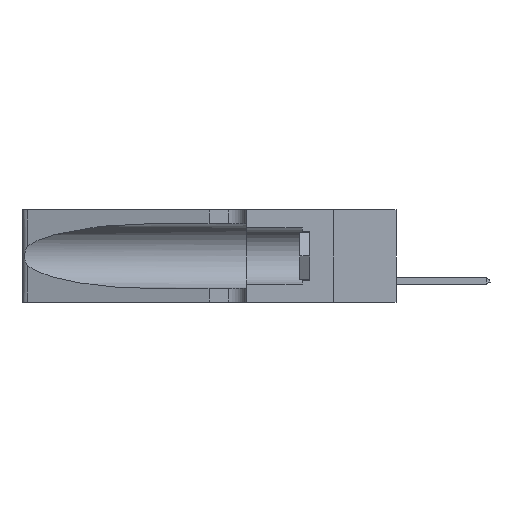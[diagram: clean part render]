
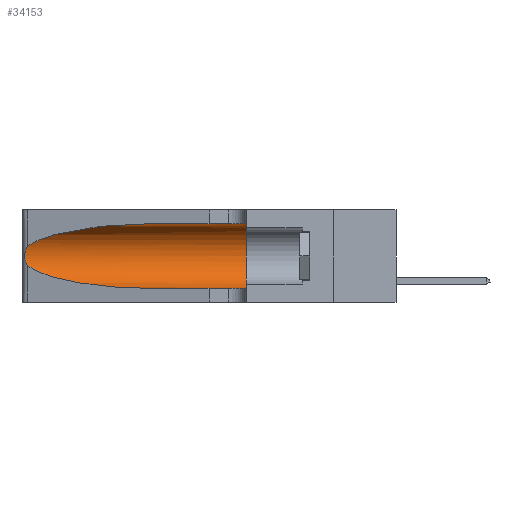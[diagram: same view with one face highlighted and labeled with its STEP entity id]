
A CAD part, left-side view. The second image highlights one B-rep face of the part: STEP entity #34153.
In plain terms, the highlighted cylindrical face has radius 3.308 mm (diameter 6.617 mm), a partial arc.
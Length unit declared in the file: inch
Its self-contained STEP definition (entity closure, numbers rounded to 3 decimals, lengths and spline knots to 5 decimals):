
#397 = EDGE_CURVE ( 'NONE', #566, #38153, #36444, .T. ) ;
#566 = VERTEX_POINT ( 'NONE', #9797 ) ;
#2162 = CARTESIAN_POINT ( 'NONE',  ( 0.25789, 1.23486, 0.15765 ) ) ;
#2301 = CARTESIAN_POINT ( 'NONE',  ( 0.2373, 1.15595, 0.08982 ) ) ;
#2417 = CARTESIAN_POINT ( 'NONE',  ( 0.25487, 1.22718, 0.22369 ) ) ;
#2835 = EDGE_CURVE ( 'NONE', #3416, #7719, #19045, .T. ) ;
#3194 = ORIENTED_EDGE ( 'NONE', *, *, #2835, .T. ) ;
#3416 = VERTEX_POINT ( 'NONE', #14175 ) ;
#3968 = ORIENTED_EDGE ( 'NONE', *, *, #397, .T. ) ;
#4473 = DIRECTION ( 'NONE',  ( 0., -1., 0. ) ) ;
#5065 = CARTESIAN_POINT ( 'NONE',  ( 0.25856, 1.23593, 0.16098 ) ) ;
#5157 = EDGE_CURVE ( 'NONE', #25724, #7719, #25460, .T. ) ;
#6444 = VERTEX_POINT ( 'NONE', #20930 ) ;
#6486 =( BOUNDED_CURVE ( )  B_SPLINE_CURVE ( 3, ( #29626, #2301, #23371, #26388 ),
 .UNSPECIFIED., .F., .T. ) 
 B_SPLINE_CURVE_WITH_KNOTS ( ( 4, 4 ),
 ( 3.44316, 4.71239 ),
 .UNSPECIFIED. ) 
 CURVE ( )  GEOMETRIC_REPRESENTATION_ITEM ( )  RATIONAL_B_SPLINE_CURVE ( ( 1., 0.87, 0.87, 1. ) ) 
 REPRESENTATION_ITEM ( '' )  );
#7080 = EDGE_CURVE ( 'NONE', #38153, #3416, #6486, .T. ) ;
#7719 = VERTEX_POINT ( 'NONE', #26398 ) ;
#7881 = CARTESIAN_POINT ( 'NONE',  ( 0.1305, 0.72297, 0.31525 ) ) ;
#8062 = CARTESIAN_POINT ( 'NONE',  ( 0.25639, 1.23184, 0.21858 ) ) ;
#9599 = DIRECTION ( 'NONE',  ( 0., -1., 0. ) ) ;
#9710 = AXIS2_PLACEMENT_3D ( 'NONE', #32426, #23690, #35901 ) ;
#9797 = CARTESIAN_POINT ( 'NONE',  ( 0.25487, 1.22718, 0.22369 ) ) ;
#10760 = CARTESIAN_POINT ( 'NONE',  ( 0.25787, 1.23484, 0.2124 ) ) ;
#11286 = CARTESIAN_POINT ( 'NONE',  ( 0.25555, 1.22994, 0.2215 ) ) ;
#13149 = CARTESIAN_POINT ( 'NONE',  ( 0.1305, 1.61858, 0.31525 ) ) ;
#13601 = EDGE_LOOP ( 'NONE', ( #15380, #3968, #37531, #3194, #24132, #28954 ) ) ;
#13895 = CARTESIAN_POINT ( 'NONE',  ( 0.25487, 1.22718, 0.22369 ) ) ;
#14175 = CARTESIAN_POINT ( 'NONE',  ( 0.1305, 0.72297, 0.05475 ) ) ;
#15380 = ORIENTED_EDGE ( 'NONE', *, *, #20780, .T. ) ;
#15802 = AXIS2_PLACEMENT_3D ( 'NONE', #28276, #4473, #25434 ) ;
#16767 = VECTOR ( 'NONE', #37063, 39.37008 ) ;
#16968 = CARTESIAN_POINT ( 'NONE',  ( 0.25639, 1.23186, 0.15144 ) ) ;
#17222 = CARTESIAN_POINT ( 'NONE',  ( 0.26075, 1.23896, 0.178 ) ) ;
#18327 = FACE_OUTER_BOUND ( 'NONE', #13601, .T. ) ;
#19045 = LINE ( 'NONE', #27676, #33085 ) ;
#19806 = CYLINDRICAL_SURFACE ( 'NONE', #15802, 0.13025 ) ;
#19819 = CARTESIAN_POINT ( 'NONE',  ( 0.26018, 1.23835, 0.19895 ) ) ;
#19952 = CARTESIAN_POINT ( 'NONE',  ( 0.25555, 1.22993, 0.14849 ) ) ;
#20355 = CARTESIAN_POINT ( 'NONE',  ( 0.25487, 1.22718, 0.14631 ) ) ;
#20780 = EDGE_CURVE ( 'NONE', #6444, #566, #30728, .T. ) ;
#20921 = CARTESIAN_POINT ( 'NONE',  ( 0.25487, 1.22718, 0.14631 ) ) ;
#20930 = CARTESIAN_POINT ( 'NONE',  ( 0.1305, 0.72297, 0.31525 ) ) ;
#21660 = EDGE_CURVE ( 'NONE', #6444, #25724, #27024, .T. ) ;
#22451 = CARTESIAN_POINT ( 'NONE',  ( 0.1305, 0.35, 0.31525 ) ) ;
#22968 = CARTESIAN_POINT ( 'NONE',  ( 0.26075, 1.23896, 0.19203 ) ) ;
#23189 = CARTESIAN_POINT ( 'NONE',  ( 0.2373, 1.15595, 0.28018 ) ) ;
#23371 = CARTESIAN_POINT ( 'NONE',  ( 0.18966, 0.96281, 0.05475 ) ) ;
#23690 = DIRECTION ( 'NONE',  ( 0., 1., 0. ) ) ;
#24132 = ORIENTED_EDGE ( 'NONE', *, *, #5157, .F. ) ;
#25434 = DIRECTION ( 'NONE',  ( 0., 0., -1. ) ) ;
#25460 = CIRCLE ( 'NONE', #9710, 0.13025 ) ;
#25724 = VERTEX_POINT ( 'NONE', #22451 ) ;
#26388 = CARTESIAN_POINT ( 'NONE',  ( 0.1305, 0.72297, 0.05475 ) ) ;
#26398 = CARTESIAN_POINT ( 'NONE',  ( 0.1305, 0.35, 0.05475 ) ) ;
#27024 = LINE ( 'NONE', #13149, #16767 ) ;
#27676 = CARTESIAN_POINT ( 'NONE',  ( 0.1305, 1.61858, 0.05475 ) ) ;
#28276 = CARTESIAN_POINT ( 'NONE',  ( 0.1305, 1.61858, 0.185 ) ) ;
#28812 = CARTESIAN_POINT ( 'NONE',  ( 0.18966, 0.96281, 0.31525 ) ) ;
#28954 = ORIENTED_EDGE ( 'NONE', *, *, #21660, .F. ) ;
#29626 = CARTESIAN_POINT ( 'NONE',  ( 0.25487, 1.22718, 0.14631 ) ) ;
#30728 =( BOUNDED_CURVE ( )  B_SPLINE_CURVE ( 3, ( #7881, #28812, #23189, #13895 ),
 .UNSPECIFIED., .F., .F. ) 
 B_SPLINE_CURVE_WITH_KNOTS ( ( 4, 4 ),
 ( 1.5708, 2.84003 ),
 .UNSPECIFIED. ) 
 CURVE ( )  GEOMETRIC_REPRESENTATION_ITEM ( )  RATIONAL_B_SPLINE_CURVE ( ( 1., 0.87, 0.87, 1. ) ) 
 REPRESENTATION_ITEM ( '' )  );
#32098 = CARTESIAN_POINT ( 'NONE',  ( 0.25854, 1.2359, 0.20912 ) ) ;
#32228 = CARTESIAN_POINT ( 'NONE',  ( 0.26017, 1.23833, 0.17102 ) ) ;
#32426 = CARTESIAN_POINT ( 'NONE',  ( 0.1305, 0.35, 0.185 ) ) ;
#33085 = VECTOR ( 'NONE', #9599, 39.37008 ) ;
#34153 = ADVANCED_FACE ( 'NONE', ( #18327 ), #19806, .F. ) ;
#35901 = DIRECTION ( 'NONE',  ( 0., 0., 1. ) ) ;
#36444 = B_SPLINE_CURVE_WITH_KNOTS ( 'NONE', 3,
 ( #2417, #11286, #8062, #10760, #32098, #19819, #22968, #17222, #32228, #5065, #2162, #16968, #19952, #20355 ),
 .UNSPECIFIED., .F., .F.,
 ( 4, 2, 2, 2, 2, 2, 4 ),
 ( 0., 0.00027, 0.00053, 0.00107, 0.0016, 0.00187, 0.00214 ),
 .UNSPECIFIED. ) ;
#37063 = DIRECTION ( 'NONE',  ( 0., -1., 0. ) ) ;
#37531 = ORIENTED_EDGE ( 'NONE', *, *, #7080, .T. ) ;
#38153 = VERTEX_POINT ( 'NONE', #20921 ) ;
